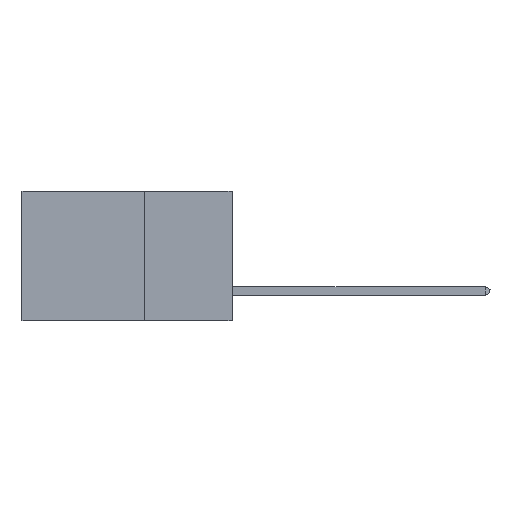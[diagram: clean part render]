
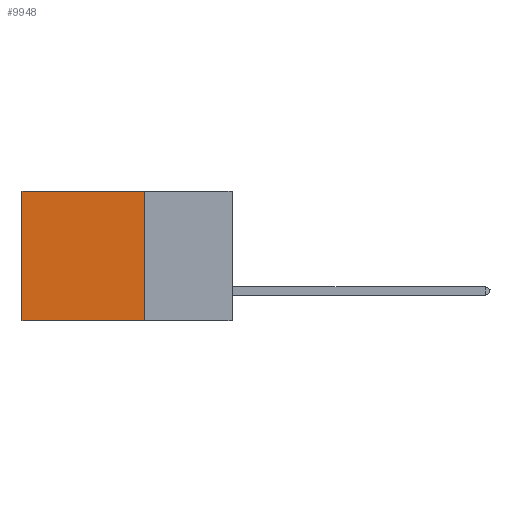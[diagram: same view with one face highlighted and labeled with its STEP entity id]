
A CAD part, left-side view. The second image highlights one B-rep face of the part: STEP entity #9948.
In plain terms, the highlighted planar face has unit normal (-1, 0, 0).
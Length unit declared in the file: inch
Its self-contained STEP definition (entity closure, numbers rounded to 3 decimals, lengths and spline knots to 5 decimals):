
#1953 = CARTESIAN_POINT ( 'NONE',  ( 0.2875, 0.25, 0. ) ) ;
#3803 = CARTESIAN_POINT ( 'NONE',  ( 0.2875, 0.25, 0. ) ) ;
#4233 = LINE ( 'NONE', #22920, #32872 ) ;
#4689 = VERTEX_POINT ( 'NONE', #31260 ) ;
#5500 = DIRECTION ( 'NONE',  ( 0., 1., 0. ) ) ;
#6960 = EDGE_CURVE ( 'NONE', #16656, #19662, #33766, .T. ) ;
#7461 = DIRECTION ( 'NONE',  ( 0., 0., -1. ) ) ;
#7646 = DIRECTION ( 'NONE',  ( 0., 1., 0. ) ) ;
#8186 = CARTESIAN_POINT ( 'NONE',  ( 0.2875, 0.6, 0. ) ) ;
#9948 = ADVANCED_FACE ( 'NONE', ( #18790 ), #34324, .F. ) ;
#10926 = EDGE_CURVE ( 'NONE', #19662, #30670, #32093, .T. ) ;
#15267 = CARTESIAN_POINT ( 'NONE',  ( 0.2875, 0.25, 0. ) ) ;
#15544 = ORIENTED_EDGE ( 'NONE', *, *, #19236, .F. ) ;
#16656 = VERTEX_POINT ( 'NONE', #3803 ) ;
#18180 = ORIENTED_EDGE ( 'NONE', *, *, #23690, .F. ) ;
#18790 = FACE_OUTER_BOUND ( 'NONE', #30917, .T. ) ;
#19187 = AXIS2_PLACEMENT_3D ( 'NONE', #36596, #27555, #27823 ) ;
#19236 = EDGE_CURVE ( 'NONE', #4689, #30670, #4233, .T. ) ;
#19662 = VERTEX_POINT ( 'NONE', #28501 ) ;
#19995 = ORIENTED_EDGE ( 'NONE', *, *, #6960, .T. ) ;
#20840 = DIRECTION ( 'NONE',  ( 0., 0., -1. ) ) ;
#22418 = ORIENTED_EDGE ( 'NONE', *, *, #10926, .T. ) ;
#22920 = CARTESIAN_POINT ( 'NONE',  ( 0.2875, 0.25, -0.37 ) ) ;
#23690 = EDGE_CURVE ( 'NONE', #16656, #4689, #32078, .T. ) ;
#25010 = VECTOR ( 'NONE', #7646, 39.37008 ) ;
#27555 = DIRECTION ( 'NONE',  ( 1., 0., 0. ) ) ;
#27823 = DIRECTION ( 'NONE',  ( 0., 0., -1. ) ) ;
#28501 = CARTESIAN_POINT ( 'NONE',  ( 0.2875, 0.6, 0. ) ) ;
#30203 = VECTOR ( 'NONE', #20840, 39.37008 ) ;
#30670 = VERTEX_POINT ( 'NONE', #33118 ) ;
#30917 = EDGE_LOOP ( 'NONE', ( #22418, #15544, #18180, #19995 ) ) ;
#31260 = CARTESIAN_POINT ( 'NONE',  ( 0.2875, 0.25, -0.37 ) ) ;
#32078 = LINE ( 'NONE', #15267, #30203 ) ;
#32093 = LINE ( 'NONE', #8186, #33926 ) ;
#32872 = VECTOR ( 'NONE', #5500, 39.37008 ) ;
#33118 = CARTESIAN_POINT ( 'NONE',  ( 0.2875, 0.6, -0.37 ) ) ;
#33766 = LINE ( 'NONE', #1953, #25010 ) ;
#33926 = VECTOR ( 'NONE', #7461, 39.37008 ) ;
#34324 = PLANE ( 'NONE',  #19187 ) ;
#36596 = CARTESIAN_POINT ( 'NONE',  ( 0.2875, 0.25, 0. ) ) ;
